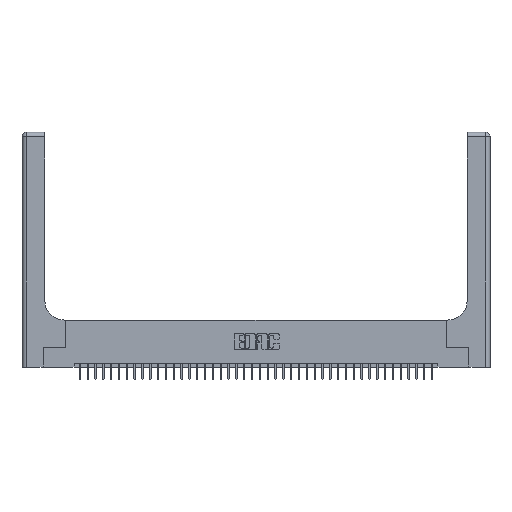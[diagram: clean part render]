
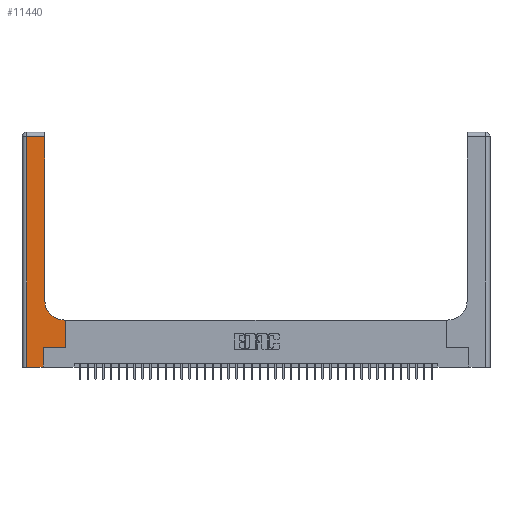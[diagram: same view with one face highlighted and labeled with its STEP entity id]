
A CAD part, top view. The second image highlights one B-rep face of the part: STEP entity #11440.
In plain terms, the highlighted planar face has unit normal (0, 0, 1).
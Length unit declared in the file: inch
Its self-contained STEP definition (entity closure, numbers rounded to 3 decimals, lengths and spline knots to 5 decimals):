
#3195 = LINE ( 'NONE', #19976, #27435 ) ;
#3673 = EDGE_CURVE ( 'NONE', #12031, #21908, #39026, .T. ) ;
#5171 = VERTEX_POINT ( 'NONE', #33295 ) ;
#5275 = VECTOR ( 'NONE', #32699, 39.37008 ) ;
#5449 = CARTESIAN_POINT ( 'NONE',  ( 0.06, 2.94, 0.37 ) ) ;
#9730 = VECTOR ( 'NONE', #17398, 39.37008 ) ;
#9860 = ORIENTED_EDGE ( 'NONE', *, *, #21630, .T. ) ;
#10936 = EDGE_CURVE ( 'NONE', #14044, #5171, #12801, .T. ) ;
#10993 = CARTESIAN_POINT ( 'NONE',  ( 0.5415, 0.85, 0.37 ) ) ;
#11440 = ADVANCED_FACE ( 'NONE', ( #20171 ), #24060, .F. ) ;
#12031 = VERTEX_POINT ( 'NONE', #27486 ) ;
#12493 = VECTOR ( 'NONE', #14178, 39.37008 ) ;
#12520 = CARTESIAN_POINT ( 'NONE',  ( 0.2915, 3., 0.37 ) ) ;
#12801 = LINE ( 'NONE', #12520, #38895 ) ;
#12956 = ORIENTED_EDGE ( 'NONE', *, *, #37721, .T. ) ;
#12968 = CARTESIAN_POINT ( 'NONE',  ( 0.5585, 0.25, 0.37 ) ) ;
#14044 = VERTEX_POINT ( 'NONE', #40707 ) ;
#14162 = DIRECTION ( 'NONE',  ( 1., 0., 0. ) ) ;
#14178 = DIRECTION ( 'NONE',  ( 0., 1., 0. ) ) ;
#14342 = ORIENTED_EDGE ( 'NONE', *, *, #35673, .T. ) ;
#15756 = EDGE_CURVE ( 'NONE', #22238, #32544, #26034, .T. ) ;
#16220 = LINE ( 'NONE', #19762, #23624 ) ;
#17398 = DIRECTION ( 'NONE',  ( 1., 0., 0. ) ) ;
#17642 = VECTOR ( 'NONE', #25984, 39.37008 ) ;
#17868 = AXIS2_PLACEMENT_3D ( 'NONE', #27094, #39844, #21030 ) ;
#19762 = CARTESIAN_POINT ( 'NONE',  ( 0.269, 0., 0.37 ) ) ;
#19767 = ORIENTED_EDGE ( 'NONE', *, *, #21745, .T. ) ;
#19904 = LINE ( 'NONE', #33044, #12493 ) ;
#19976 = CARTESIAN_POINT ( 'NONE',  ( 0., 2.94, 0.37 ) ) ;
#20107 = CARTESIAN_POINT ( 'NONE',  ( 0.2915, 0.6, 0.37 ) ) ;
#20171 = FACE_OUTER_BOUND ( 'NONE', #27294, .T. ) ;
#20582 = CARTESIAN_POINT ( 'NONE',  ( 0.269, 0.25, 0.37 ) ) ;
#21030 = DIRECTION ( 'NONE',  ( -1., 0., 0. ) ) ;
#21630 = EDGE_CURVE ( 'NONE', #33941, #22238, #23086, .T. ) ;
#21745 = EDGE_CURVE ( 'NONE', #40508, #39408, #26524, .T. ) ;
#21908 = VERTEX_POINT ( 'NONE', #37718 ) ;
#22238 = VERTEX_POINT ( 'NONE', #23669 ) ;
#23086 = LINE ( 'NONE', #23208, #5275 ) ;
#23143 = DIRECTION ( 'NONE',  ( -1., 0., 0. ) ) ;
#23208 = CARTESIAN_POINT ( 'NONE',  ( 0.06, 3., 0.37 ) ) ;
#23275 = DIRECTION ( 'NONE',  ( -1., 0., 0. ) ) ;
#23624 = VECTOR ( 'NONE', #25955, 39.37008 ) ;
#23669 = CARTESIAN_POINT ( 'NONE',  ( 0.06, 0., 0.37 ) ) ;
#24060 = PLANE ( 'NONE',  #17868 ) ;
#24467 = CARTESIAN_POINT ( 'NONE',  ( 0.269, 0.25, 0.37 ) ) ;
#25955 = DIRECTION ( 'NONE',  ( 0., 1., 0. ) ) ;
#25984 = DIRECTION ( 'NONE',  ( 1., 0., 0. ) ) ;
#26034 = LINE ( 'NONE', #38484, #17642 ) ;
#26524 = LINE ( 'NONE', #20582, #9730 ) ;
#27094 = CARTESIAN_POINT ( 'NONE',  ( 0., 3., 0.37 ) ) ;
#27294 = EDGE_LOOP ( 'NONE', ( #32530, #35469, #9860, #35001, #35513, #19767, #14342, #33116, #12956 ) ) ;
#27435 = VECTOR ( 'NONE', #23143, 39.37008 ) ;
#27453 = EDGE_CURVE ( 'NONE', #5171, #33941, #3195, .T. ) ;
#27486 = CARTESIAN_POINT ( 'NONE',  ( 0.5585, 0.6, 0.37 ) ) ;
#29355 = AXIS2_PLACEMENT_3D ( 'NONE', #10993, #33031, #14162 ) ;
#31388 = DIRECTION ( 'NONE',  ( 0., 1., 0. ) ) ;
#31401 = EDGE_CURVE ( 'NONE', #32544, #40508, #16220, .T. ) ;
#32530 = ORIENTED_EDGE ( 'NONE', *, *, #10936, .T. ) ;
#32544 = VERTEX_POINT ( 'NONE', #37694 ) ;
#32699 = DIRECTION ( 'NONE',  ( 0., -1., 0. ) ) ;
#33031 = DIRECTION ( 'NONE',  ( 0., 0., -1. ) ) ;
#33044 = CARTESIAN_POINT ( 'NONE',  ( 0.5585, 0.25, 0.37 ) ) ;
#33116 = ORIENTED_EDGE ( 'NONE', *, *, #3673, .T. ) ;
#33295 = CARTESIAN_POINT ( 'NONE',  ( 0.2915, 2.94, 0.37 ) ) ;
#33941 = VERTEX_POINT ( 'NONE', #5449 ) ;
#35001 = ORIENTED_EDGE ( 'NONE', *, *, #15756, .T. ) ;
#35469 = ORIENTED_EDGE ( 'NONE', *, *, #27453, .T. ) ;
#35513 = ORIENTED_EDGE ( 'NONE', *, *, #31401, .T. ) ;
#35673 = EDGE_CURVE ( 'NONE', #39408, #12031, #19904, .T. ) ;
#37694 = CARTESIAN_POINT ( 'NONE',  ( 0.269, 0., 0.37 ) ) ;
#37718 = CARTESIAN_POINT ( 'NONE',  ( 0.5415, 0.6, 0.37 ) ) ;
#37721 = EDGE_CURVE ( 'NONE', #21908, #14044, #38899, .T. ) ;
#38051 = VECTOR ( 'NONE', #23275, 39.37008 ) ;
#38484 = CARTESIAN_POINT ( 'NONE',  ( 0., 0., 0.37 ) ) ;
#38895 = VECTOR ( 'NONE', #31388, 39.37008 ) ;
#38899 = CIRCLE ( 'NONE', #29355, 0.25 ) ;
#39026 = LINE ( 'NONE', #20107, #38051 ) ;
#39408 = VERTEX_POINT ( 'NONE', #12968 ) ;
#39844 = DIRECTION ( 'NONE',  ( 0., 0., -1. ) ) ;
#40508 = VERTEX_POINT ( 'NONE', #24467 ) ;
#40707 = CARTESIAN_POINT ( 'NONE',  ( 0.2915, 0.85, 0.37 ) ) ;
